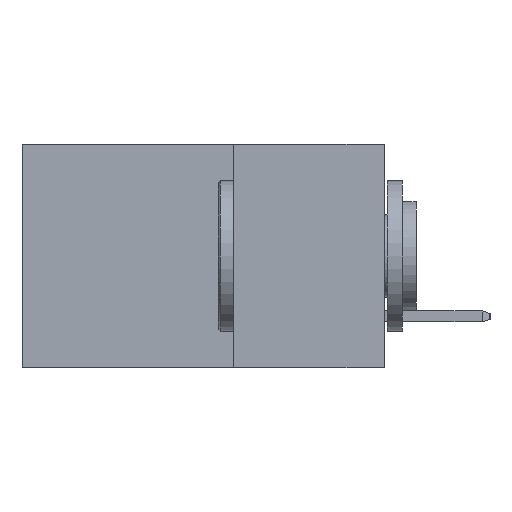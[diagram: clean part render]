
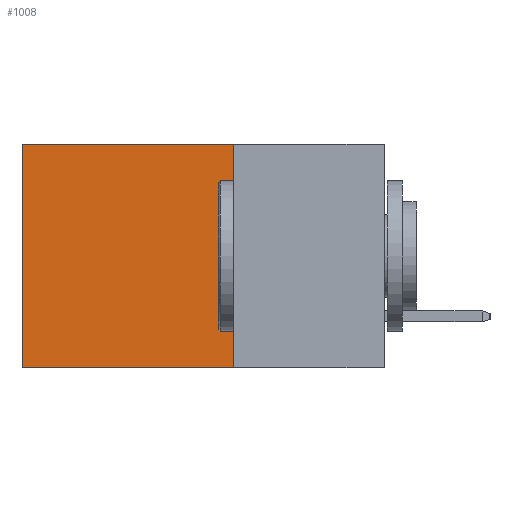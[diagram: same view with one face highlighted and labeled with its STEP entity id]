
A CAD part, left-side view. The second image highlights one B-rep face of the part: STEP entity #1008.
In plain terms, the highlighted planar face has unit normal (-1, 0, 0).
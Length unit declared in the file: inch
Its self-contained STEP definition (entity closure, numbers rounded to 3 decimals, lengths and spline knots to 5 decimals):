
#112 = AXIS2_PLACEMENT_3D ( 'NONE', #2763, #13718, #1287 ) ;
#386 = EDGE_LOOP ( 'NONE', ( #13710, #7757, #13156, #14230 ) ) ;
#1008 = ADVANCED_FACE ( 'NONE', ( #9953 ), #1563, .F. ) ;
#1138 = CARTESIAN_POINT ( 'NONE',  ( 0.2615, 0.25, 0. ) ) ;
#1287 = DIRECTION ( 'NONE',  ( 0., 0., -1. ) ) ;
#1563 = PLANE ( 'NONE',  #112 ) ;
#1725 = DIRECTION ( 'NONE',  ( 0., 0., -1. ) ) ;
#2543 = DIRECTION ( 'NONE',  ( 0., 1., 0. ) ) ;
#2763 = CARTESIAN_POINT ( 'NONE',  ( 0.2615, 0.25, -0.37 ) ) ;
#2794 = VERTEX_POINT ( 'NONE', #11566 ) ;
#3706 = EDGE_CURVE ( 'NONE', #2794, #4377, #14183, .T. ) ;
#4377 = VERTEX_POINT ( 'NONE', #7552 ) ;
#7552 = CARTESIAN_POINT ( 'NONE',  ( 0.2615, 0.25, -0.37 ) ) ;
#7757 = ORIENTED_EDGE ( 'NONE', *, *, #17505, .F. ) ;
#8064 = VECTOR ( 'NONE', #1725, 39.37008 ) ;
#8113 = VERTEX_POINT ( 'NONE', #16714 ) ;
#8476 = LINE ( 'NONE', #11349, #8064 ) ;
#9390 = CARTESIAN_POINT ( 'NONE',  ( 0.2615, 0.25, -0.37 ) ) ;
#9782 = DIRECTION ( 'NONE',  ( 0., 0., -1. ) ) ;
#9953 = FACE_OUTER_BOUND ( 'NONE', #386, .T. ) ;
#11263 = VERTEX_POINT ( 'NONE', #12063 ) ;
#11290 = CARTESIAN_POINT ( 'NONE',  ( 0.2615, 0.25, -0.37 ) ) ;
#11337 = EDGE_CURVE ( 'NONE', #2794, #11263, #13378, .T. ) ;
#11349 = CARTESIAN_POINT ( 'NONE',  ( 0.2615, 0.6, -0.37 ) ) ;
#11566 = CARTESIAN_POINT ( 'NONE',  ( 0.2615, 0.25, 0. ) ) ;
#12063 = CARTESIAN_POINT ( 'NONE',  ( 0.2615, 0.6, 0. ) ) ;
#12130 = VECTOR ( 'NONE', #12693, 39.37008 ) ;
#12693 = DIRECTION ( 'NONE',  ( 0., 1., 0. ) ) ;
#13156 = ORIENTED_EDGE ( 'NONE', *, *, #3706, .F. ) ;
#13378 = LINE ( 'NONE', #1138, #16490 ) ;
#13710 = ORIENTED_EDGE ( 'NONE', *, *, #17532, .T. ) ;
#13718 = DIRECTION ( 'NONE',  ( 1., 0., 0. ) ) ;
#14183 = LINE ( 'NONE', #9390, #15439 ) ;
#14230 = ORIENTED_EDGE ( 'NONE', *, *, #11337, .T. ) ;
#15439 = VECTOR ( 'NONE', #9782, 39.37008 ) ;
#15705 = LINE ( 'NONE', #11290, #12130 ) ;
#16490 = VECTOR ( 'NONE', #2543, 39.37008 ) ;
#16714 = CARTESIAN_POINT ( 'NONE',  ( 0.2615, 0.6, -0.37 ) ) ;
#17505 = EDGE_CURVE ( 'NONE', #4377, #8113, #15705, .T. ) ;
#17532 = EDGE_CURVE ( 'NONE', #11263, #8113, #8476, .T. ) ;
